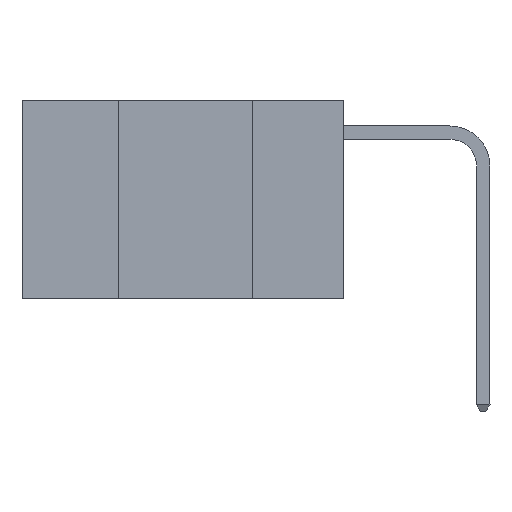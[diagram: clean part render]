
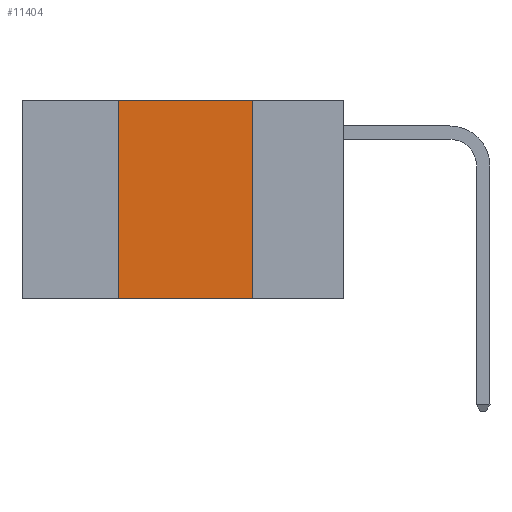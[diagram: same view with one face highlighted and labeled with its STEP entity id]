
A CAD part, left-side view. The second image highlights one B-rep face of the part: STEP entity #11404.
In plain terms, the highlighted planar face has unit normal (-1, 0, 0).
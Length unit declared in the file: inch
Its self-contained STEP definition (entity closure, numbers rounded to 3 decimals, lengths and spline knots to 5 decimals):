
#19 = DIRECTION ( 'NONE',  ( 0., 0., 1. ) ) ;
#362 = ORIENTED_EDGE ( 'NONE', *, *, #16970, .T. ) ;
#412 = CARTESIAN_POINT ( 'NONE',  ( 0., 0.42, 0. ) ) ;
#1330 = CARTESIAN_POINT ( 'NONE',  ( 0., 0.42, 0. ) ) ;
#1524 = LINE ( 'NONE', #13078, #13940 ) ;
#2559 = EDGE_LOOP ( 'NONE', ( #10832, #12335, #4892, #362 ) ) ;
#2860 = VERTEX_POINT ( 'NONE', #14181 ) ;
#2891 = CARTESIAN_POINT ( 'NONE',  ( 0., 0.42, -0.37 ) ) ;
#3920 = PLANE ( 'NONE',  #4377 ) ;
#4341 = DIRECTION ( 'NONE',  ( 0., 0., -1. ) ) ;
#4377 = AXIS2_PLACEMENT_3D ( 'NONE', #15604, #16801, #7661 ) ;
#4854 = VERTEX_POINT ( 'NONE', #2891 ) ;
#4892 = ORIENTED_EDGE ( 'NONE', *, *, #8660, .F. ) ;
#5275 = VERTEX_POINT ( 'NONE', #412 ) ;
#5466 = VECTOR ( 'NONE', #4341, 39.37008 ) ;
#5505 = CARTESIAN_POINT ( 'NONE',  ( 0., 0.17, -0.37 ) ) ;
#5681 = DIRECTION ( 'NONE',  ( 0., -1., 0. ) ) ;
#6410 = LINE ( 'NONE', #1330, #14196 ) ;
#6460 = LINE ( 'NONE', #11744, #5466 ) ;
#7661 = DIRECTION ( 'NONE',  ( 0., 0., -1. ) ) ;
#8295 = VECTOR ( 'NONE', #5681, 39.37008 ) ;
#8660 = EDGE_CURVE ( 'NONE', #4854, #5275, #6410, .T. ) ;
#8961 = FACE_OUTER_BOUND ( 'NONE', #2559, .T. ) ;
#9516 = EDGE_CURVE ( 'NONE', #5275, #2860, #1524, .T. ) ;
#10748 = CARTESIAN_POINT ( 'NONE',  ( 0., 0.6, -0.37 ) ) ;
#10832 = ORIENTED_EDGE ( 'NONE', *, *, #11466, .F. ) ;
#10913 = LINE ( 'NONE', #10748, #8295 ) ;
#11404 = ADVANCED_FACE ( 'NONE', ( #8961 ), #3920, .F. ) ;
#11466 = EDGE_CURVE ( 'NONE', #2860, #15111, #6460, .T. ) ;
#11744 = CARTESIAN_POINT ( 'NONE',  ( 0., 0.17, 0. ) ) ;
#12335 = ORIENTED_EDGE ( 'NONE', *, *, #9516, .F. ) ;
#13078 = CARTESIAN_POINT ( 'NONE',  ( 0., 0.6, 0. ) ) ;
#13940 = VECTOR ( 'NONE', #14712, 39.37008 ) ;
#14181 = CARTESIAN_POINT ( 'NONE',  ( 0., 0.17, 0. ) ) ;
#14196 = VECTOR ( 'NONE', #19, 39.37008 ) ;
#14712 = DIRECTION ( 'NONE',  ( 0., -1., 0. ) ) ;
#15111 = VERTEX_POINT ( 'NONE', #5505 ) ;
#15604 = CARTESIAN_POINT ( 'NONE',  ( 0., 0.6, 0. ) ) ;
#16801 = DIRECTION ( 'NONE',  ( 1., 0., 0. ) ) ;
#16970 = EDGE_CURVE ( 'NONE', #4854, #15111, #10913, .T. ) ;
